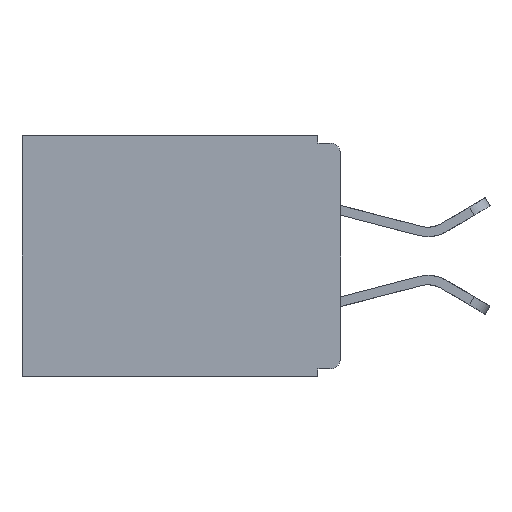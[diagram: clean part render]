
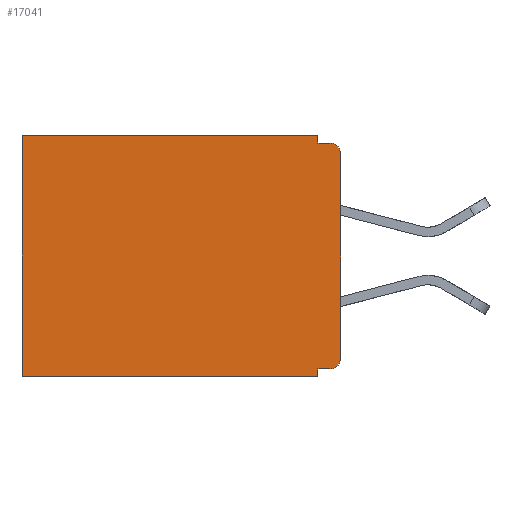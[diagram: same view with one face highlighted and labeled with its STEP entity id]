
A CAD part, left-side view. The second image highlights one B-rep face of the part: STEP entity #17041.
In plain terms, the highlighted planar face has unit normal (-1, 0, 0).
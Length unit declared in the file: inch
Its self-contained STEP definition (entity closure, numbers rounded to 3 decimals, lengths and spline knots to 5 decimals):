
#131 = LINE ( 'NONE', #3552, #25442 ) ;
#159 = LINE ( 'NONE', #5573, #31075 ) ;
#422 = AXIS2_PLACEMENT_3D ( 'NONE', #26282, #11714, #28730 ) ;
#551 = EDGE_LOOP ( 'NONE', ( #1978, #1983, #15889, #29537, #14520, #31055, #24596, #20150, #26349, #23559 ) ) ;
#972 = DIRECTION ( 'NONE',  ( -1., 0., 0. ) ) ;
#1251 = CARTESIAN_POINT ( 'NONE',  ( 0.3, 0., 0. ) ) ;
#1427 = CARTESIAN_POINT ( 'NONE',  ( 0.3, 0., -0.33 ) ) ;
#1459 = VERTEX_POINT ( 'NONE', #4344 ) ;
#1582 = VERTEX_POINT ( 'NONE', #27971 ) ;
#1686 = EDGE_CURVE ( 'NONE', #1582, #11314, #5915, .T. ) ;
#1978 = ORIENTED_EDGE ( 'NONE', *, *, #24918, .F. ) ;
#1983 = ORIENTED_EDGE ( 'NONE', *, *, #26910, .T. ) ;
#2229 = VECTOR ( 'NONE', #19556, 39.37008 ) ;
#2697 = VECTOR ( 'NONE', #30234, 39.37008 ) ;
#2996 = LINE ( 'NONE', #14886, #2229 ) ;
#3306 = FACE_OUTER_BOUND ( 'NONE', #551, .T. ) ;
#3552 = CARTESIAN_POINT ( 'NONE',  ( 0.3, 0.031, 0. ) ) ;
#3836 = VERTEX_POINT ( 'NONE', #8076 ) ;
#4344 = CARTESIAN_POINT ( 'NONE',  ( 0.3, 0.031, 0. ) ) ;
#5043 = LINE ( 'NONE', #6041, #23800 ) ;
#5573 = CARTESIAN_POINT ( 'NONE',  ( 0.3, 0.031, -0.33 ) ) ;
#5915 = LINE ( 'NONE', #1427, #31028 ) ;
#6041 = CARTESIAN_POINT ( 'NONE',  ( 0.3, 0., -0.01 ) ) ;
#6963 = LINE ( 'NONE', #1251, #14277 ) ;
#7624 = VERTEX_POINT ( 'NONE', #26050 ) ;
#8076 = CARTESIAN_POINT ( 'NONE',  ( 0.3, 0.015, -0.01 ) ) ;
#9778 = VERTEX_POINT ( 'NONE', #14760 ) ;
#10086 = LINE ( 'NONE', #15692, #2697 ) ;
#10358 = EDGE_CURVE ( 'NONE', #1459, #7624, #131, .T. ) ;
#10565 = DIRECTION ( 'NONE',  ( 0., 0., -1. ) ) ;
#10578 = DIRECTION ( 'NONE',  ( 0., 0., -1. ) ) ;
#10603 = PLANE ( 'NONE',  #21768 ) ;
#11314 = VERTEX_POINT ( 'NONE', #29142 ) ;
#11714 = DIRECTION ( 'NONE',  ( -1., 0., 0. ) ) ;
#11966 = VERTEX_POINT ( 'NONE', #27328 ) ;
#12510 = VECTOR ( 'NONE', #10578, 39.37008 ) ;
#12636 = EDGE_CURVE ( 'NONE', #11966, #1582, #159, .T. ) ;
#13039 = CARTESIAN_POINT ( 'NONE',  ( 0.3, 0., -0.33 ) ) ;
#13083 = EDGE_CURVE ( 'NONE', #9778, #11314, #26208, .T. ) ;
#13490 = DIRECTION ( 'NONE',  ( 0., -1., 0. ) ) ;
#13828 = CARTESIAN_POINT ( 'NONE',  ( 0.3, 0., -0.305 ) ) ;
#14277 = VECTOR ( 'NONE', #23366, 39.37008 ) ;
#14497 = EDGE_CURVE ( 'NONE', #7624, #3836, #5043, .T. ) ;
#14520 = ORIENTED_EDGE ( 'NONE', *, *, #20349, .T. ) ;
#14760 = CARTESIAN_POINT ( 'NONE',  ( 0.3, 0.437, 0. ) ) ;
#14886 = CARTESIAN_POINT ( 'NONE',  ( 0.3, 0., -0.33 ) ) ;
#15054 = VERTEX_POINT ( 'NONE', #15579 ) ;
#15503 = DIRECTION ( 'NONE',  ( 0., 0., -1. ) ) ;
#15579 = CARTESIAN_POINT ( 'NONE',  ( 0.3, 0., -0.025 ) ) ;
#15581 = CIRCLE ( 'NONE', #19999, 0.015 ) ;
#15692 = CARTESIAN_POINT ( 'NONE',  ( 0.3, 0., -0.32 ) ) ;
#15741 = CARTESIAN_POINT ( 'NONE',  ( 0.3, 0.015, -0.025 ) ) ;
#15889 = ORIENTED_EDGE ( 'NONE', *, *, #14497, .F. ) ;
#17041 = ADVANCED_FACE ( 'NONE', ( #3306 ), #10603, .F. ) ;
#18162 = DIRECTION ( 'NONE',  ( 0., 0., -1. ) ) ;
#18750 = VERTEX_POINT ( 'NONE', #19482 ) ;
#19232 = EDGE_CURVE ( 'NONE', #18750, #23333, #19987, .T. ) ;
#19482 = CARTESIAN_POINT ( 'NONE',  ( 0.3, 0.015, -0.32 ) ) ;
#19556 = DIRECTION ( 'NONE',  ( 0., 0., -1. ) ) ;
#19987 = CIRCLE ( 'NONE', #422, 0.015 ) ;
#19999 = AXIS2_PLACEMENT_3D ( 'NONE', #15741, #972, #18162 ) ;
#20150 = ORIENTED_EDGE ( 'NONE', *, *, #12636, .F. ) ;
#20266 = EDGE_CURVE ( 'NONE', #18750, #11966, #10086, .T. ) ;
#20349 = EDGE_CURVE ( 'NONE', #1459, #9778, #6963, .T. ) ;
#20697 = DIRECTION ( 'NONE',  ( 0., 0., -1. ) ) ;
#21768 = AXIS2_PLACEMENT_3D ( 'NONE', #13039, #30042, #15503 ) ;
#23333 = VERTEX_POINT ( 'NONE', #13828 ) ;
#23366 = DIRECTION ( 'NONE',  ( 0., 1., 0. ) ) ;
#23559 = ORIENTED_EDGE ( 'NONE', *, *, #19232, .T. ) ;
#23800 = VECTOR ( 'NONE', #13490, 39.37008 ) ;
#24596 = ORIENTED_EDGE ( 'NONE', *, *, #1686, .F. ) ;
#24918 = EDGE_CURVE ( 'NONE', #15054, #23333, #2996, .T. ) ;
#25148 = CARTESIAN_POINT ( 'NONE',  ( 0.3, 0.437, -0.33 ) ) ;
#25442 = VECTOR ( 'NONE', #20697, 39.37008 ) ;
#26050 = CARTESIAN_POINT ( 'NONE',  ( 0.3, 0.031, -0.01 ) ) ;
#26208 = LINE ( 'NONE', #25148, #12510 ) ;
#26282 = CARTESIAN_POINT ( 'NONE',  ( 0.3, 0.015, -0.305 ) ) ;
#26349 = ORIENTED_EDGE ( 'NONE', *, *, #20266, .F. ) ;
#26910 = EDGE_CURVE ( 'NONE', #15054, #3836, #15581, .T. ) ;
#27328 = CARTESIAN_POINT ( 'NONE',  ( 0.3, 0.031, -0.32 ) ) ;
#27971 = CARTESIAN_POINT ( 'NONE',  ( 0.3, 0.031, -0.33 ) ) ;
#28730 = DIRECTION ( 'NONE',  ( 0., 0., -1. ) ) ;
#29142 = CARTESIAN_POINT ( 'NONE',  ( 0.3, 0.437, -0.33 ) ) ;
#29537 = ORIENTED_EDGE ( 'NONE', *, *, #10358, .F. ) ;
#30042 = DIRECTION ( 'NONE',  ( 1., 0., 0. ) ) ;
#30234 = DIRECTION ( 'NONE',  ( 0., 1., 0. ) ) ;
#31028 = VECTOR ( 'NONE', #31478, 39.37008 ) ;
#31055 = ORIENTED_EDGE ( 'NONE', *, *, #13083, .T. ) ;
#31075 = VECTOR ( 'NONE', #10565, 39.37008 ) ;
#31478 = DIRECTION ( 'NONE',  ( 0., 1., 0. ) ) ;
